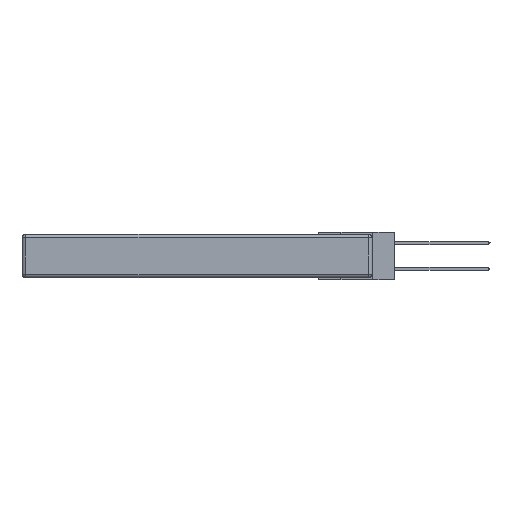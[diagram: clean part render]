
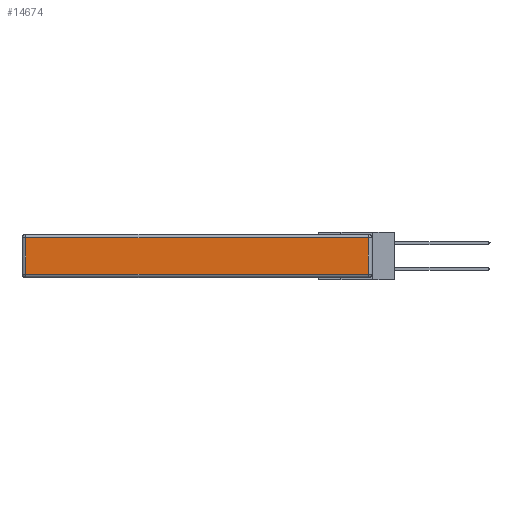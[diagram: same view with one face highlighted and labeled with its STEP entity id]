
A CAD part, left-side view. The second image highlights one B-rep face of the part: STEP entity #14674.
In plain terms, the highlighted planar face has unit normal (-1, 0, 0).
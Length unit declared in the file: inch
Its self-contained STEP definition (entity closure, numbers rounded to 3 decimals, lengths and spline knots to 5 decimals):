
#1180 = CARTESIAN_POINT ( 'NONE',  ( 0., 0.03, -0.343 ) ) ;
#1526 = ORIENTED_EDGE ( 'NONE', *, *, #12496, .T. ) ;
#3058 = EDGE_LOOP ( 'NONE', ( #1526, #8258, #16825, #6367 ) ) ;
#3181 = DIRECTION ( 'NONE',  ( 0., 0., 1. ) ) ;
#4584 = VERTEX_POINT ( 'NONE', #16446 ) ;
#4840 = DIRECTION ( 'NONE',  ( 0., -1., 0. ) ) ;
#6189 = CARTESIAN_POINT ( 'NONE',  ( 0., 0.03, -0.03 ) ) ;
#6367 = ORIENTED_EDGE ( 'NONE', *, *, #21598, .T. ) ;
#6528 = EDGE_CURVE ( 'NONE', #14729, #24532, #12384, .T. ) ;
#6766 = CARTESIAN_POINT ( 'NONE',  ( 0., 0., -0.313 ) ) ;
#7069 = VECTOR ( 'NONE', #10745, 39.37008 ) ;
#8197 = AXIS2_PLACEMENT_3D ( 'NONE', #15955, #19851, #9949 ) ;
#8258 = ORIENTED_EDGE ( 'NONE', *, *, #20393, .T. ) ;
#8311 = CARTESIAN_POINT ( 'NONE',  ( 0., 2.72, -0.03 ) ) ;
#9165 = VECTOR ( 'NONE', #14600, 39.37008 ) ;
#9856 = PLANE ( 'NONE',  #8197 ) ;
#9949 = DIRECTION ( 'NONE',  ( 0., 0., 1. ) ) ;
#10745 = DIRECTION ( 'NONE',  ( 0., 1., 0. ) ) ;
#11736 = VECTOR ( 'NONE', #4840, 39.37008 ) ;
#12384 = LINE ( 'NONE', #16687, #7069 ) ;
#12496 = EDGE_CURVE ( 'NONE', #4584, #14588, #14867, .T. ) ;
#13297 = LINE ( 'NONE', #1180, #18839 ) ;
#14588 = VERTEX_POINT ( 'NONE', #15431 ) ;
#14600 = DIRECTION ( 'NONE',  ( 0., 0., -1. ) ) ;
#14674 = ADVANCED_FACE ( 'NONE', ( #25126 ), #9856, .T. ) ;
#14729 = VERTEX_POINT ( 'NONE', #6189 ) ;
#14867 = LINE ( 'NONE', #6766, #11736 ) ;
#15431 = CARTESIAN_POINT ( 'NONE',  ( 0., 0.03, -0.313 ) ) ;
#15955 = CARTESIAN_POINT ( 'NONE',  ( 0., 0., -0.343 ) ) ;
#16446 = CARTESIAN_POINT ( 'NONE',  ( 0., 2.72, -0.313 ) ) ;
#16687 = CARTESIAN_POINT ( 'NONE',  ( 0., 2.75, -0.03 ) ) ;
#16825 = ORIENTED_EDGE ( 'NONE', *, *, #6528, .T. ) ;
#18839 = VECTOR ( 'NONE', #3181, 39.37008 ) ;
#19132 = LINE ( 'NONE', #23391, #9165 ) ;
#19851 = DIRECTION ( 'NONE',  ( -1., 0., 0. ) ) ;
#20393 = EDGE_CURVE ( 'NONE', #14588, #14729, #13297, .T. ) ;
#21598 = EDGE_CURVE ( 'NONE', #24532, #4584, #19132, .T. ) ;
#23391 = CARTESIAN_POINT ( 'NONE',  ( 0., 2.72, -0.343 ) ) ;
#24532 = VERTEX_POINT ( 'NONE', #8311 ) ;
#25126 = FACE_OUTER_BOUND ( 'NONE', #3058, .T. ) ;
